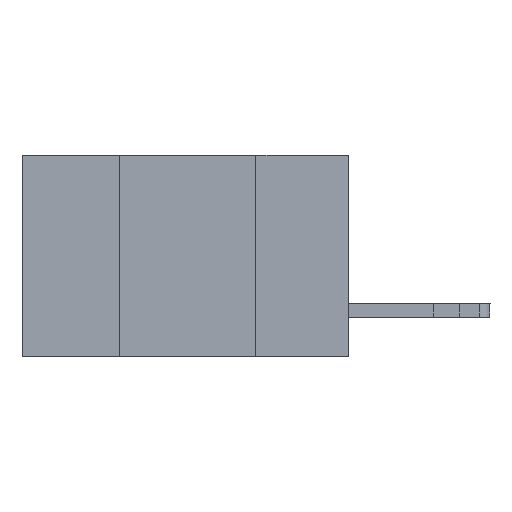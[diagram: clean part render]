
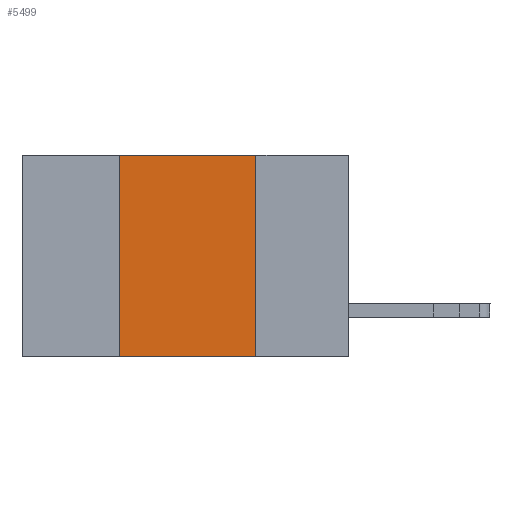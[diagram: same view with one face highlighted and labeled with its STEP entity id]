
A CAD part, left-side view. The second image highlights one B-rep face of the part: STEP entity #5499.
In plain terms, the highlighted planar face has unit normal (-1, 0, 0).
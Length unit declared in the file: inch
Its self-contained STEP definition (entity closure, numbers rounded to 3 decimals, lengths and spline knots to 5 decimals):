
#28 = LINE ( 'NONE', #5902, #7099 ) ;
#190 = CARTESIAN_POINT ( 'NONE',  ( 0., 0.42, 0. ) ) ;
#688 = CARTESIAN_POINT ( 'NONE',  ( 0., 0.6, -0.37 ) ) ;
#696 = DIRECTION ( 'NONE',  ( 1., 0., 0. ) ) ;
#1158 = CARTESIAN_POINT ( 'NONE',  ( 0., 0.17, -0.37 ) ) ;
#1292 = VECTOR ( 'NONE', #5294, 39.37008 ) ;
#1949 = VECTOR ( 'NONE', #2248, 39.37008 ) ;
#2248 = DIRECTION ( 'NONE',  ( 0., -1., 0. ) ) ;
#2678 = ORIENTED_EDGE ( 'NONE', *, *, #17826, .F. ) ;
#3688 = CARTESIAN_POINT ( 'NONE',  ( 0., 0.6, 0. ) ) ;
#4817 = CARTESIAN_POINT ( 'NONE',  ( 0., 0.6, 0. ) ) ;
#4873 = CARTESIAN_POINT ( 'NONE',  ( 0., 0.42, -0.37 ) ) ;
#5294 = DIRECTION ( 'NONE',  ( 0., -1., 0. ) ) ;
#5482 = DIRECTION ( 'NONE',  ( 0., 0., 1. ) ) ;
#5499 = ADVANCED_FACE ( 'NONE', ( #12052 ), #16743, .F. ) ;
#5592 = LINE ( 'NONE', #3688, #1949 ) ;
#5902 = CARTESIAN_POINT ( 'NONE',  ( 0., 0.17, 0. ) ) ;
#6539 = ORIENTED_EDGE ( 'NONE', *, *, #9395, .F. ) ;
#6828 = LINE ( 'NONE', #688, #1292 ) ;
#7099 = VECTOR ( 'NONE', #8514, 39.37008 ) ;
#7434 = VECTOR ( 'NONE', #5482, 39.37008 ) ;
#8205 = AXIS2_PLACEMENT_3D ( 'NONE', #4817, #696, #9451 ) ;
#8398 = ORIENTED_EDGE ( 'NONE', *, *, #10117, .T. ) ;
#8514 = DIRECTION ( 'NONE',  ( 0., 0., -1. ) ) ;
#8996 = VERTEX_POINT ( 'NONE', #1158 ) ;
#9395 = EDGE_CURVE ( 'NONE', #10213, #8996, #28, .T. ) ;
#9451 = DIRECTION ( 'NONE',  ( 0., 0., -1. ) ) ;
#10117 = EDGE_CURVE ( 'NONE', #18456, #8996, #6828, .T. ) ;
#10190 = EDGE_CURVE ( 'NONE', #18456, #11148, #13080, .T. ) ;
#10213 = VERTEX_POINT ( 'NONE', #15766 ) ;
#11148 = VERTEX_POINT ( 'NONE', #190 ) ;
#11445 = CARTESIAN_POINT ( 'NONE',  ( 0., 0.42, 0. ) ) ;
#12052 = FACE_OUTER_BOUND ( 'NONE', #18654, .T. ) ;
#12577 = ORIENTED_EDGE ( 'NONE', *, *, #10190, .F. ) ;
#13080 = LINE ( 'NONE', #11445, #7434 ) ;
#15766 = CARTESIAN_POINT ( 'NONE',  ( 0., 0.17, 0. ) ) ;
#16743 = PLANE ( 'NONE',  #8205 ) ;
#17826 = EDGE_CURVE ( 'NONE', #11148, #10213, #5592, .T. ) ;
#18456 = VERTEX_POINT ( 'NONE', #4873 ) ;
#18654 = EDGE_LOOP ( 'NONE', ( #6539, #2678, #12577, #8398 ) ) ;
